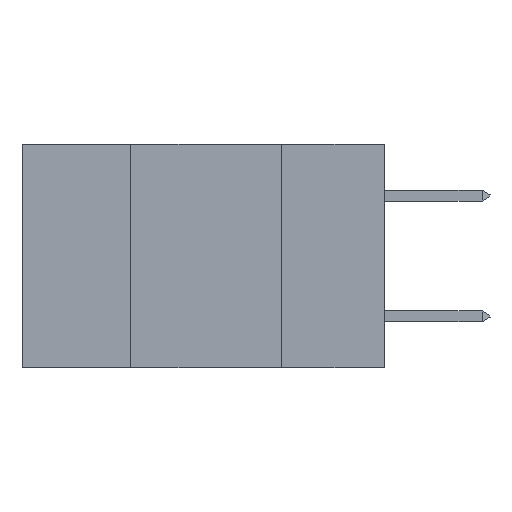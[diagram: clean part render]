
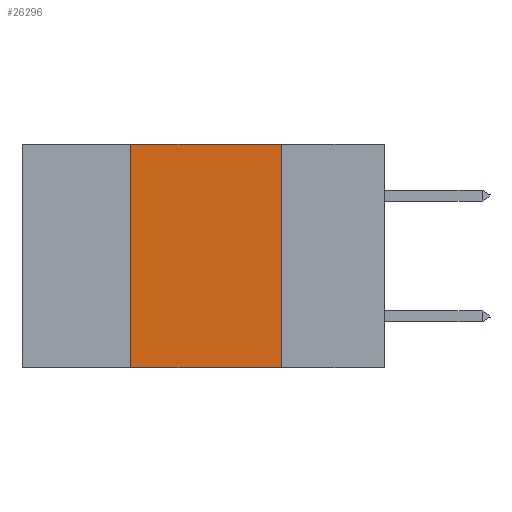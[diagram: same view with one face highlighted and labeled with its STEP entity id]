
A CAD part, left-side view. The second image highlights one B-rep face of the part: STEP entity #26296.
In plain terms, the highlighted planar face has unit normal (-1, 0, 0).
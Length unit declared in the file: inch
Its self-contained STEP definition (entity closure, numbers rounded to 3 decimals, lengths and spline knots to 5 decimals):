
#1608 = DIRECTION ( 'NONE',  ( 0., -1., 0. ) ) ;
#1952 = CARTESIAN_POINT ( 'NONE',  ( 0., 0.42, 0. ) ) ;
#2911 = DIRECTION ( 'NONE',  ( 0., 0., 1. ) ) ;
#4303 = CARTESIAN_POINT ( 'NONE',  ( 0., 0.6, 0. ) ) ;
#6859 = DIRECTION ( 'NONE',  ( 1., 0., 0. ) ) ;
#7856 = CARTESIAN_POINT ( 'NONE',  ( 0., 0.6, 0. ) ) ;
#8195 = VERTEX_POINT ( 'NONE', #1952 ) ;
#9992 = DIRECTION ( 'NONE',  ( 0., -1., 0. ) ) ;
#12021 = VECTOR ( 'NONE', #2911, 39.37008 ) ;
#12293 = ORIENTED_EDGE ( 'NONE', *, *, #16355, .F. ) ;
#12861 = CARTESIAN_POINT ( 'NONE',  ( 0., 0.42, 0. ) ) ;
#15780 = ORIENTED_EDGE ( 'NONE', *, *, #20467, .F. ) ;
#16355 = EDGE_CURVE ( 'NONE', #27075, #8195, #36134, .T. ) ;
#16757 = LINE ( 'NONE', #32511, #17658 ) ;
#17558 = CARTESIAN_POINT ( 'NONE',  ( 0., 0.17, 0. ) ) ;
#17658 = VECTOR ( 'NONE', #9992, 39.37008 ) ;
#18255 = EDGE_CURVE ( 'NONE', #8195, #29617, #27929, .T. ) ;
#18557 = VECTOR ( 'NONE', #21397, 39.37008 ) ;
#19003 = ORIENTED_EDGE ( 'NONE', *, *, #20510, .T. ) ;
#20467 = EDGE_CURVE ( 'NONE', #29617, #34588, #24456, .T. ) ;
#20476 = ORIENTED_EDGE ( 'NONE', *, *, #18255, .F. ) ;
#20510 = EDGE_CURVE ( 'NONE', #27075, #34588, #16757, .T. ) ;
#21171 = DIRECTION ( 'NONE',  ( 0., 0., -1. ) ) ;
#21397 = DIRECTION ( 'NONE',  ( 0., 0., -1. ) ) ;
#22270 = CARTESIAN_POINT ( 'NONE',  ( 0., 0.42, -0.37 ) ) ;
#24456 = LINE ( 'NONE', #30095, #18557 ) ;
#24650 = PLANE ( 'NONE',  #28561 ) ;
#26296 = ADVANCED_FACE ( 'NONE', ( #37196 ), #24650, .F. ) ;
#27075 = VERTEX_POINT ( 'NONE', #22270 ) ;
#27437 = VECTOR ( 'NONE', #1608, 39.37008 ) ;
#27929 = LINE ( 'NONE', #7856, #27437 ) ;
#28473 = CARTESIAN_POINT ( 'NONE',  ( 0., 0.17, -0.37 ) ) ;
#28561 = AXIS2_PLACEMENT_3D ( 'NONE', #4303, #6859, #21171 ) ;
#28903 = EDGE_LOOP ( 'NONE', ( #15780, #20476, #12293, #19003 ) ) ;
#29617 = VERTEX_POINT ( 'NONE', #17558 ) ;
#30095 = CARTESIAN_POINT ( 'NONE',  ( 0., 0.17, 0. ) ) ;
#32511 = CARTESIAN_POINT ( 'NONE',  ( 0., 0.6, -0.37 ) ) ;
#34588 = VERTEX_POINT ( 'NONE', #28473 ) ;
#36134 = LINE ( 'NONE', #12861, #12021 ) ;
#37196 = FACE_OUTER_BOUND ( 'NONE', #28903, .T. ) ;
